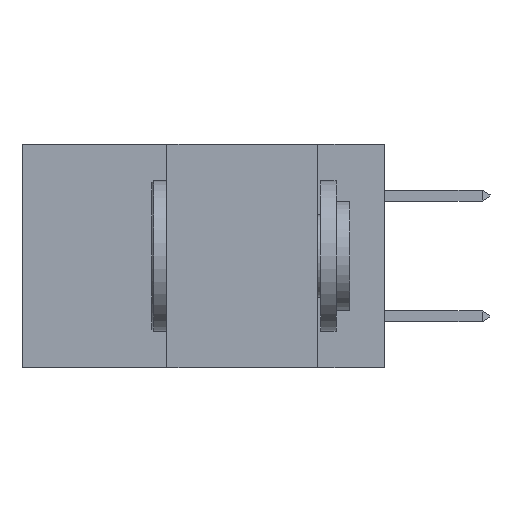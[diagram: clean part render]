
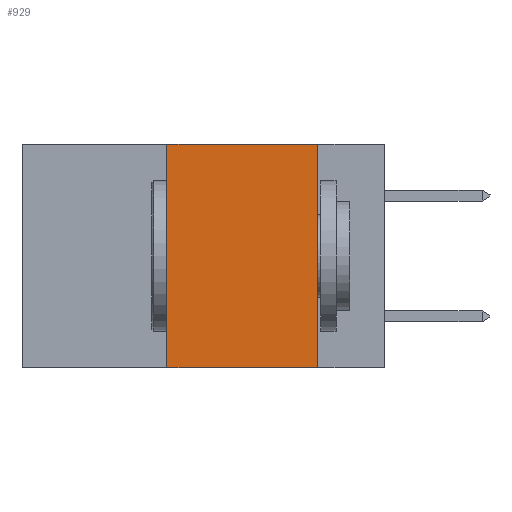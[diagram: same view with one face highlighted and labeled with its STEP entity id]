
A CAD part, left-side view. The second image highlights one B-rep face of the part: STEP entity #929.
In plain terms, the highlighted planar face has unit normal (-1, 0, 0).
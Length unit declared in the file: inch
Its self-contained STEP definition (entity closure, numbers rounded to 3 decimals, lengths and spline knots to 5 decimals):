
#370 = VECTOR ( 'NONE', #10137, 39.37008 ) ;
#867 = ORIENTED_EDGE ( 'NONE', *, *, #5929, .T. ) ;
#929 = ADVANCED_FACE ( 'NONE', ( #4102 ), #5824, .F. ) ;
#1448 = LINE ( 'NONE', #14824, #13865 ) ;
#1631 = LINE ( 'NONE', #14494, #5060 ) ;
#2989 = DIRECTION ( 'NONE',  ( 0., 0., -1. ) ) ;
#3325 = DIRECTION ( 'NONE',  ( 1., 0., 0. ) ) ;
#3585 = CARTESIAN_POINT ( 'NONE',  ( 0., 0.6, 0. ) ) ;
#3953 = LINE ( 'NONE', #7710, #370 ) ;
#4102 = FACE_OUTER_BOUND ( 'NONE', #5254, .T. ) ;
#5060 = VECTOR ( 'NONE', #6324, 39.37008 ) ;
#5254 = EDGE_LOOP ( 'NONE', ( #7253, #7368, #8138, #867 ) ) ;
#5824 = PLANE ( 'NONE',  #12574 ) ;
#5878 = CARTESIAN_POINT ( 'NONE',  ( 0., 0.6, -0.37 ) ) ;
#5929 = EDGE_CURVE ( 'NONE', #11403, #11446, #10864, .T. ) ;
#6324 = DIRECTION ( 'NONE',  ( 0., 0., -1. ) ) ;
#6721 = EDGE_CURVE ( 'NONE', #11403, #15460, #1448, .T. ) ;
#7253 = ORIENTED_EDGE ( 'NONE', *, *, #12253, .F. ) ;
#7368 = ORIENTED_EDGE ( 'NONE', *, *, #13798, .F. ) ;
#7710 = CARTESIAN_POINT ( 'NONE',  ( 0., 0.6, 0. ) ) ;
#8138 = ORIENTED_EDGE ( 'NONE', *, *, #6721, .F. ) ;
#9392 = CARTESIAN_POINT ( 'NONE',  ( 0., 0.36, -0.37 ) ) ;
#10137 = DIRECTION ( 'NONE',  ( 0., -1., 0. ) ) ;
#10864 = LINE ( 'NONE', #5878, #13543 ) ;
#11387 = DIRECTION ( 'NONE',  ( 0., -1., 0. ) ) ;
#11403 = VERTEX_POINT ( 'NONE', #9392 ) ;
#11446 = VERTEX_POINT ( 'NONE', #11781 ) ;
#11781 = CARTESIAN_POINT ( 'NONE',  ( 0., 0.11, -0.37 ) ) ;
#11959 = CARTESIAN_POINT ( 'NONE',  ( 0., 0.11, 0. ) ) ;
#12253 = EDGE_CURVE ( 'NONE', #15395, #11446, #1631, .T. ) ;
#12574 = AXIS2_PLACEMENT_3D ( 'NONE', #3585, #3325, #2989 ) ;
#13543 = VECTOR ( 'NONE', #11387, 39.37008 ) ;
#13798 = EDGE_CURVE ( 'NONE', #15460, #15395, #3953, .T. ) ;
#13865 = VECTOR ( 'NONE', #14195, 39.37008 ) ;
#14195 = DIRECTION ( 'NONE',  ( 0., 0., 1. ) ) ;
#14345 = CARTESIAN_POINT ( 'NONE',  ( 0., 0.36, 0. ) ) ;
#14494 = CARTESIAN_POINT ( 'NONE',  ( 0., 0.11, 0. ) ) ;
#14824 = CARTESIAN_POINT ( 'NONE',  ( 0., 0.36, 0. ) ) ;
#15395 = VERTEX_POINT ( 'NONE', #11959 ) ;
#15460 = VERTEX_POINT ( 'NONE', #14345 ) ;
